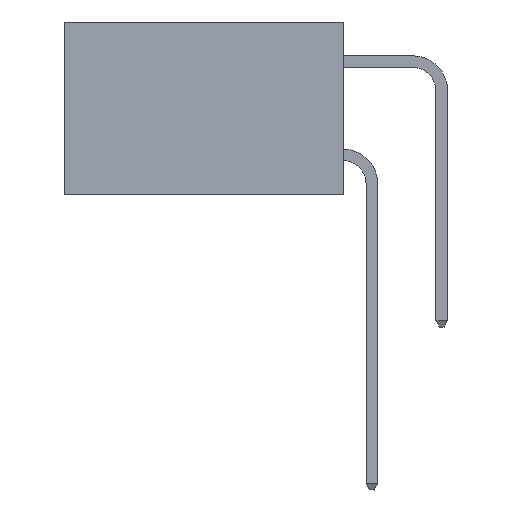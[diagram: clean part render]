
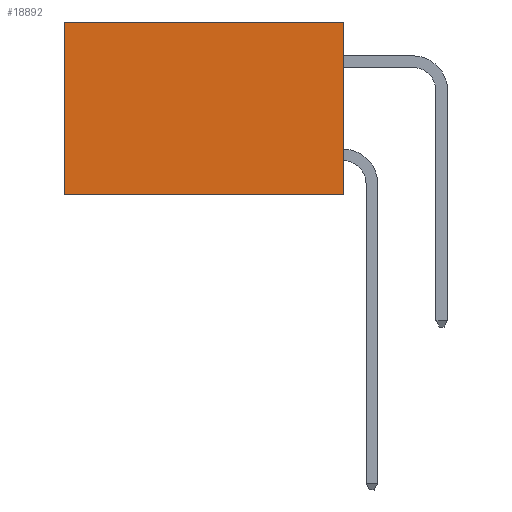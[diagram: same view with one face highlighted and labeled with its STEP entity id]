
A CAD part, left-side view. The second image highlights one B-rep face of the part: STEP entity #18892.
In plain terms, the highlighted planar face has unit normal (-1, 0, 0).
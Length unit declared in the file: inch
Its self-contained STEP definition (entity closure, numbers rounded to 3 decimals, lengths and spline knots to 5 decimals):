
#655 = ORIENTED_EDGE ( 'NONE', *, *, #12258, .T. ) ;
#799 = ORIENTED_EDGE ( 'NONE', *, *, #16758, .T. ) ;
#1420 = VERTEX_POINT ( 'NONE', #23739 ) ;
#5557 = DIRECTION ( 'NONE',  ( 0., 1., 0. ) ) ;
#5616 = ORIENTED_EDGE ( 'NONE', *, *, #14706, .F. ) ;
#5737 = VECTOR ( 'NONE', #24328, 39.37008 ) ;
#6417 = EDGE_LOOP ( 'NONE', ( #655, #5616, #18606, #799 ) ) ;
#7152 = EDGE_CURVE ( 'NONE', #1420, #16234, #7221, .T. ) ;
#7221 = LINE ( 'NONE', #25758, #26469 ) ;
#9347 = LINE ( 'NONE', #21970, #5737 ) ;
#9531 = VECTOR ( 'NONE', #15892, 39.37008 ) ;
#9929 = FACE_OUTER_BOUND ( 'NONE', #6417, .T. ) ;
#11763 = CARTESIAN_POINT ( 'NONE',  ( 0.298, 0., 0. ) ) ;
#12113 = CARTESIAN_POINT ( 'NONE',  ( 0.298, 0.6, -0.37 ) ) ;
#12258 = EDGE_CURVE ( 'NONE', #16341, #13520, #9347, .T. ) ;
#13520 = VERTEX_POINT ( 'NONE', #12113 ) ;
#14706 = EDGE_CURVE ( 'NONE', #16234, #13520, #16047, .T. ) ;
#15064 = AXIS2_PLACEMENT_3D ( 'NONE', #17036, #25431, #18935 ) ;
#15892 = DIRECTION ( 'NONE',  ( 0., 1., 0. ) ) ;
#16047 = LINE ( 'NONE', #22176, #9531 ) ;
#16234 = VERTEX_POINT ( 'NONE', #23666 ) ;
#16341 = VERTEX_POINT ( 'NONE', #24627 ) ;
#16758 = EDGE_CURVE ( 'NONE', #1420, #16341, #19475, .T. ) ;
#16857 = PLANE ( 'NONE',  #15064 ) ;
#17036 = CARTESIAN_POINT ( 'NONE',  ( 0.298, 0., 0. ) ) ;
#18606 = ORIENTED_EDGE ( 'NONE', *, *, #7152, .F. ) ;
#18892 = ADVANCED_FACE ( 'NONE', ( #9929 ), #16857, .F. ) ;
#18935 = DIRECTION ( 'NONE',  ( 0., 0., -1. ) ) ;
#19475 = LINE ( 'NONE', #11763, #24361 ) ;
#21970 = CARTESIAN_POINT ( 'NONE',  ( 0.298, 0.6, 0. ) ) ;
#22176 = CARTESIAN_POINT ( 'NONE',  ( 0.298, 0., -0.37 ) ) ;
#23666 = CARTESIAN_POINT ( 'NONE',  ( 0.298, 0., -0.37 ) ) ;
#23739 = CARTESIAN_POINT ( 'NONE',  ( 0.298, 0., 0. ) ) ;
#24328 = DIRECTION ( 'NONE',  ( 0., 0., -1. ) ) ;
#24361 = VECTOR ( 'NONE', #5557, 39.37008 ) ;
#24627 = CARTESIAN_POINT ( 'NONE',  ( 0.298, 0.6, 0. ) ) ;
#25431 = DIRECTION ( 'NONE',  ( 1., 0., 0. ) ) ;
#25758 = CARTESIAN_POINT ( 'NONE',  ( 0.298, 0., 0. ) ) ;
#25844 = DIRECTION ( 'NONE',  ( 0., 0., -1. ) ) ;
#26469 = VECTOR ( 'NONE', #25844, 39.37008 ) ;
